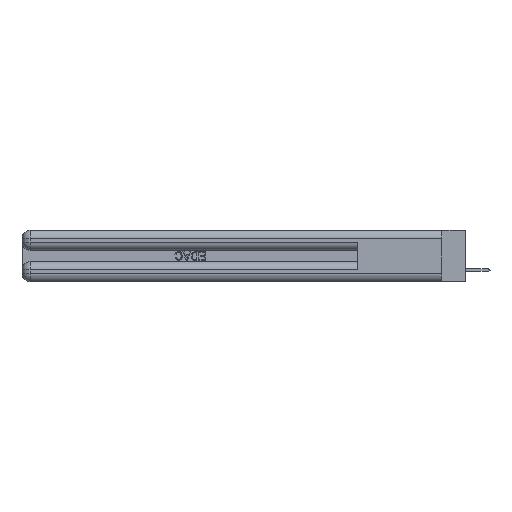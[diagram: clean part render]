
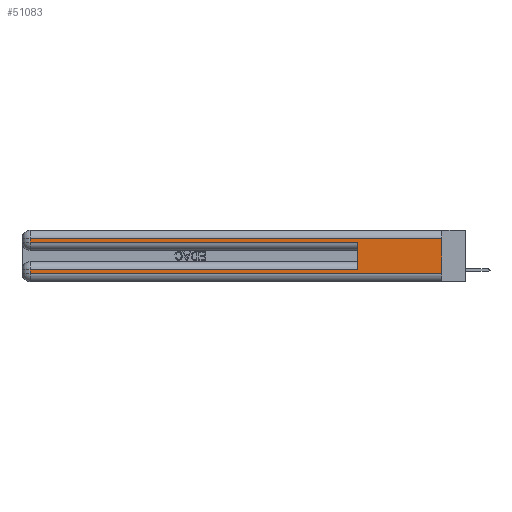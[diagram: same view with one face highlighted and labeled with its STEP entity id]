
A CAD part, left-side view. The second image highlights one B-rep face of the part: STEP entity #51083.
In plain terms, the highlighted planar face has unit normal (-1, 0, 0).
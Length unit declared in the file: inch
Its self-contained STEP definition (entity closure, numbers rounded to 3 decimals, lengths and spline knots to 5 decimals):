
#956 = LINE ( 'NONE', #24752, #42814 ) ;
#1120 = CARTESIAN_POINT ( 'NONE',  ( 0., 2.94, 0.085 ) ) ;
#3746 = ORIENTED_EDGE ( 'NONE', *, *, #39683, .T. ) ;
#3966 = DIRECTION ( 'NONE',  ( 0., -1., 0. ) ) ;
#4187 = VERTEX_POINT ( 'NONE', #1120 ) ;
#4515 = VECTOR ( 'NONE', #19648, 39.37008 ) ;
#4842 = EDGE_CURVE ( 'NONE', #12953, #33984, #21670, .T. ) ;
#5870 = CARTESIAN_POINT ( 'NONE',  ( 0., 2.94, 0.285 ) ) ;
#6427 = VECTOR ( 'NONE', #12975, 39.37008 ) ;
#7159 = VECTOR ( 'NONE', #11882, 39.37008 ) ;
#9532 = DIRECTION ( 'NONE',  ( 0., 0., -1. ) ) ;
#10681 = ORIENTED_EDGE ( 'NONE', *, *, #4842, .T. ) ;
#11132 = VERTEX_POINT ( 'NONE', #30988 ) ;
#11882 = DIRECTION ( 'NONE',  ( 0., 0., -1. ) ) ;
#12322 = LINE ( 'NONE', #34853, #45418 ) ;
#12468 = CARTESIAN_POINT ( 'NONE',  ( 0., 0.6, 0.145 ) ) ;
#12953 = VERTEX_POINT ( 'NONE', #39370 ) ;
#12975 = DIRECTION ( 'NONE',  ( 0., 0., -1. ) ) ;
#13164 = LINE ( 'NONE', #12468, #27740 ) ;
#13500 = DIRECTION ( 'NONE',  ( 0., -1., 0. ) ) ;
#14626 = CARTESIAN_POINT ( 'NONE',  ( 0., 2.94, 0.37 ) ) ;
#15626 = EDGE_CURVE ( 'NONE', #4187, #20266, #25038, .T. ) ;
#15865 = CARTESIAN_POINT ( 'NONE',  ( 0., 2.94, 0.06 ) ) ;
#16026 = EDGE_CURVE ( 'NONE', #33984, #49451, #956, .T. ) ;
#16113 = CARTESIAN_POINT ( 'NONE',  ( 0., 0., 0.31 ) ) ;
#16824 = LINE ( 'NONE', #49119, #42568 ) ;
#16856 = EDGE_CURVE ( 'NONE', #33288, #39195, #12322, .T. ) ;
#19648 = DIRECTION ( 'NONE',  ( 0., 1., 0. ) ) ;
#20266 = VERTEX_POINT ( 'NONE', #15865 ) ;
#20999 = CARTESIAN_POINT ( 'NONE',  ( 0., 0., 0.06 ) ) ;
#21670 = LINE ( 'NONE', #46438, #7159 ) ;
#22657 = CARTESIAN_POINT ( 'NONE',  ( 0., 0., 0.06 ) ) ;
#22963 = EDGE_CURVE ( 'NONE', #11132, #49451, #13164, .T. ) ;
#23078 = CARTESIAN_POINT ( 'NONE',  ( 0., 0.6, 0.285 ) ) ;
#24752 = CARTESIAN_POINT ( 'NONE',  ( 0., 0., 0.285 ) ) ;
#24837 = ORIENTED_EDGE ( 'NONE', *, *, #32854, .T. ) ;
#25038 = LINE ( 'NONE', #14626, #6427 ) ;
#27740 = VECTOR ( 'NONE', #50802, 39.37008 ) ;
#29139 = ORIENTED_EDGE ( 'NONE', *, *, #16026, .T. ) ;
#29287 = EDGE_LOOP ( 'NONE', ( #34504, #29828, #10681, #29139, #43225, #24837, #39954, #3746 ) ) ;
#29828 = ORIENTED_EDGE ( 'NONE', *, *, #40286, .T. ) ;
#30988 = CARTESIAN_POINT ( 'NONE',  ( 0., 0.6, 0.085 ) ) ;
#31422 = PLANE ( 'NONE',  #32377 ) ;
#31991 = DIRECTION ( 'NONE',  ( 1., 0., 0. ) ) ;
#32377 = AXIS2_PLACEMENT_3D ( 'NONE', #48083, #31991, #35860 ) ;
#32854 = EDGE_CURVE ( 'NONE', #11132, #4187, #50939, .T. ) ;
#33288 = VERTEX_POINT ( 'NONE', #16113 ) ;
#33984 = VERTEX_POINT ( 'NONE', #5870 ) ;
#34504 = ORIENTED_EDGE ( 'NONE', *, *, #16856, .F. ) ;
#34853 = CARTESIAN_POINT ( 'NONE',  ( 0., 0., 0.37 ) ) ;
#35860 = DIRECTION ( 'NONE',  ( 0., 0., -1. ) ) ;
#36462 = CARTESIAN_POINT ( 'NONE',  ( 0., 0., 0.085 ) ) ;
#39195 = VERTEX_POINT ( 'NONE', #22657 ) ;
#39370 = CARTESIAN_POINT ( 'NONE',  ( 0., 2.94, 0.31 ) ) ;
#39683 = EDGE_CURVE ( 'NONE', #20266, #39195, #51837, .T. ) ;
#39954 = ORIENTED_EDGE ( 'NONE', *, *, #15626, .T. ) ;
#40286 = EDGE_CURVE ( 'NONE', #33288, #12953, #16824, .T. ) ;
#42568 = VECTOR ( 'NONE', #44447, 39.37008 ) ;
#42814 = VECTOR ( 'NONE', #3966, 39.37008 ) ;
#43225 = ORIENTED_EDGE ( 'NONE', *, *, #22963, .F. ) ;
#44447 = DIRECTION ( 'NONE',  ( 0., 1., 0. ) ) ;
#45418 = VECTOR ( 'NONE', #9532, 39.37008 ) ;
#46438 = CARTESIAN_POINT ( 'NONE',  ( 0., 2.94, 0.37 ) ) ;
#48083 = CARTESIAN_POINT ( 'NONE',  ( 0., 0., 0.37 ) ) ;
#49119 = CARTESIAN_POINT ( 'NONE',  ( 0., 0., 0.31 ) ) ;
#49451 = VERTEX_POINT ( 'NONE', #23078 ) ;
#50802 = DIRECTION ( 'NONE',  ( 0., 0., 1. ) ) ;
#50939 = LINE ( 'NONE', #36462, #4515 ) ;
#51083 = ADVANCED_FACE ( 'NONE', ( #53791 ), #31422, .F. ) ;
#51837 = LINE ( 'NONE', #20999, #53859 ) ;
#53791 = FACE_OUTER_BOUND ( 'NONE', #29287, .T. ) ;
#53859 = VECTOR ( 'NONE', #13500, 39.37008 ) ;
